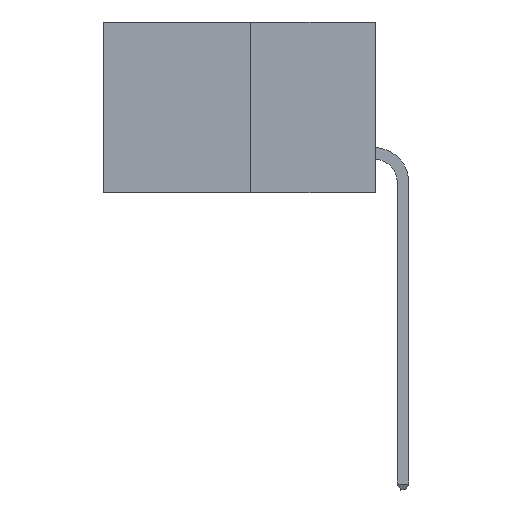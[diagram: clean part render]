
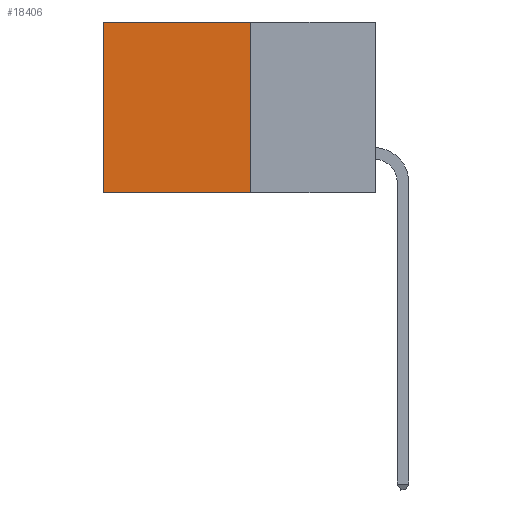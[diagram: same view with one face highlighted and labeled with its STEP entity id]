
A CAD part, left-side view. The second image highlights one B-rep face of the part: STEP entity #18406.
In plain terms, the highlighted planar face has unit normal (-1, 0, 0).
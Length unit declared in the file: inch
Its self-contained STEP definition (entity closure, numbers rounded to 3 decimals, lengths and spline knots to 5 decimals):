
#3199 = PLANE ( 'NONE',  #30039 ) ;
#4106 = EDGE_CURVE ( 'NONE', #9725, #22326, #13533, .T. ) ;
#4157 = DIRECTION ( 'NONE',  ( 0., 0., -1. ) ) ;
#4415 = DIRECTION ( 'NONE',  ( 0., 1., 0. ) ) ;
#4855 = VECTOR ( 'NONE', #23239, 39.37008 ) ;
#5631 = CARTESIAN_POINT ( 'NONE',  ( 0.277, 0.27, -0.37 ) ) ;
#6506 = CARTESIAN_POINT ( 'NONE',  ( 0.277, 0.27, -0.37 ) ) ;
#7154 = CARTESIAN_POINT ( 'NONE',  ( 0.277, 0.59, 0. ) ) ;
#8094 = DIRECTION ( 'NONE',  ( 1., 0., 0. ) ) ;
#8693 = CARTESIAN_POINT ( 'NONE',  ( 0.277, 0.27, 0. ) ) ;
#9321 = CARTESIAN_POINT ( 'NONE',  ( 0.277, 0.59, -0.37 ) ) ;
#9725 = VERTEX_POINT ( 'NONE', #23219 ) ;
#11379 = LINE ( 'NONE', #8693, #4855 ) ;
#11707 = LINE ( 'NONE', #9321, #30236 ) ;
#11781 = ORIENTED_EDGE ( 'NONE', *, *, #4106, .F. ) ;
#12374 = EDGE_CURVE ( 'NONE', #25010, #22326, #11707, .T. ) ;
#13078 = ORIENTED_EDGE ( 'NONE', *, *, #30976, .T. ) ;
#13533 = LINE ( 'NONE', #25147, #19202 ) ;
#14099 = EDGE_CURVE ( 'NONE', #25605, #9725, #22187, .T. ) ;
#15741 = VECTOR ( 'NONE', #4157, 39.37008 ) ;
#18406 = ADVANCED_FACE ( 'NONE', ( #23068 ), #3199, .F. ) ;
#19202 = VECTOR ( 'NONE', #4415, 39.37008 ) ;
#21992 = ORIENTED_EDGE ( 'NONE', *, *, #12374, .T. ) ;
#22187 = LINE ( 'NONE', #6506, #15741 ) ;
#22326 = VERTEX_POINT ( 'NONE', #31117 ) ;
#23068 = FACE_OUTER_BOUND ( 'NONE', #25322, .T. ) ;
#23219 = CARTESIAN_POINT ( 'NONE',  ( 0.277, 0.27, -0.37 ) ) ;
#23239 = DIRECTION ( 'NONE',  ( 0., 1., 0. ) ) ;
#23266 = CARTESIAN_POINT ( 'NONE',  ( 0.277, 0.27, 0. ) ) ;
#23885 = DIRECTION ( 'NONE',  ( 0., 0., -1. ) ) ;
#25010 = VERTEX_POINT ( 'NONE', #7154 ) ;
#25114 = DIRECTION ( 'NONE',  ( 0., 0., -1. ) ) ;
#25147 = CARTESIAN_POINT ( 'NONE',  ( 0.277, 0.27, -0.37 ) ) ;
#25322 = EDGE_LOOP ( 'NONE', ( #21992, #11781, #30872, #13078 ) ) ;
#25605 = VERTEX_POINT ( 'NONE', #23266 ) ;
#30039 = AXIS2_PLACEMENT_3D ( 'NONE', #5631, #8094, #25114 ) ;
#30236 = VECTOR ( 'NONE', #23885, 39.37008 ) ;
#30872 = ORIENTED_EDGE ( 'NONE', *, *, #14099, .F. ) ;
#30976 = EDGE_CURVE ( 'NONE', #25605, #25010, #11379, .T. ) ;
#31117 = CARTESIAN_POINT ( 'NONE',  ( 0.277, 0.59, -0.37 ) ) ;
